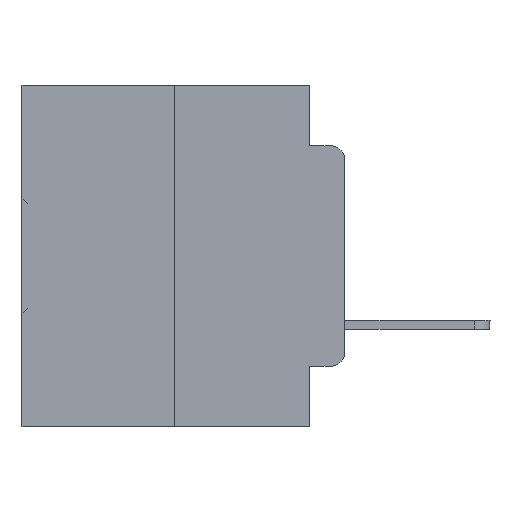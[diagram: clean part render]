
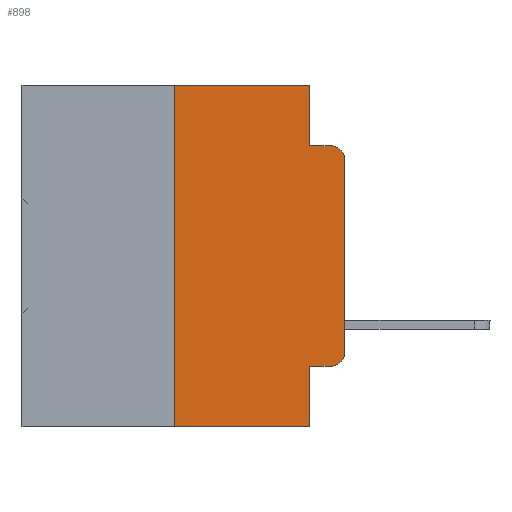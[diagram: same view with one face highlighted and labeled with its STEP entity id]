
A CAD part, left-side view. The second image highlights one B-rep face of the part: STEP entity #898.
In plain terms, the highlighted planar face has unit normal (-1, 0, 0).
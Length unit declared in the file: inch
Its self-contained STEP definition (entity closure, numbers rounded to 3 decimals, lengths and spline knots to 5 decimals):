
#272 = EDGE_CURVE ( 'NONE', #18981, #21185, #23101, .T. ) ;
#529 = DIRECTION ( 'NONE',  ( 0., 0., -1. ) ) ;
#868 = CARTESIAN_POINT ( 'NONE',  ( 0., 0.051, -0.4115 ) ) ;
#898 = ADVANCED_FACE ( 'NONE', ( #8043 ), #26643, .F. ) ;
#2185 = ORIENTED_EDGE ( 'NONE', *, *, #2942, .F. ) ;
#2942 = EDGE_CURVE ( 'NONE', #31427, #11571, #16630, .T. ) ;
#4294 = DIRECTION ( 'NONE',  ( 0., 0., 1. ) ) ;
#5197 = CARTESIAN_POINT ( 'NONE',  ( 0., 0.25, 0. ) ) ;
#5287 = VERTEX_POINT ( 'NONE', #15477 ) ;
#5591 = CARTESIAN_POINT ( 'NONE',  ( 0., 0.051, -0.0885 ) ) ;
#6175 = CARTESIAN_POINT ( 'NONE',  ( 0., 0., 0. ) ) ;
#6260 = LINE ( 'NONE', #33284, #33751 ) ;
#7361 = CARTESIAN_POINT ( 'NONE',  ( 0., 0.051, -0.5 ) ) ;
#7616 = EDGE_CURVE ( 'NONE', #11571, #5287, #29089, .T. ) ;
#7753 = CARTESIAN_POINT ( 'NONE',  ( 0., 0.02, -0.4115 ) ) ;
#7796 = VERTEX_POINT ( 'NONE', #28972 ) ;
#7856 = ORIENTED_EDGE ( 'NONE', *, *, #30176, .F. ) ;
#7921 = CARTESIAN_POINT ( 'NONE',  ( 0., 0.051, -0.0885 ) ) ;
#8043 = FACE_OUTER_BOUND ( 'NONE', #22246, .T. ) ;
#9012 = EDGE_CURVE ( 'NONE', #20275, #7796, #23643, .T. ) ;
#9058 = VECTOR ( 'NONE', #30257, 39.37008 ) ;
#9879 = DIRECTION ( 'NONE',  ( 0., 0., -1. ) ) ;
#9928 = CARTESIAN_POINT ( 'NONE',  ( 0., 0.25, -0.5 ) ) ;
#10040 = CARTESIAN_POINT ( 'NONE',  ( 0., 0.02, -0.1085 ) ) ;
#11191 = VERTEX_POINT ( 'NONE', #7921 ) ;
#11571 = VERTEX_POINT ( 'NONE', #5197 ) ;
#12537 = DIRECTION ( 'NONE',  ( -1., 0., 0. ) ) ;
#12617 = EDGE_CURVE ( 'NONE', #18981, #29494, #6260, .T. ) ;
#12719 = VECTOR ( 'NONE', #9879, 39.37008 ) ;
#13614 = DIRECTION ( 'NONE',  ( 0., -1., 0. ) ) ;
#14363 = DIRECTION ( 'NONE',  ( 0., 0., 1. ) ) ;
#14814 = EDGE_CURVE ( 'NONE', #29494, #20275, #16955, .T. ) ;
#15195 = DIRECTION ( 'NONE',  ( 0., 0., -1. ) ) ;
#15477 = CARTESIAN_POINT ( 'NONE',  ( 0., 0.051, 0. ) ) ;
#15895 = DIRECTION ( 'NONE',  ( 0., -1., 0. ) ) ;
#16044 = LINE ( 'NONE', #30364, #12719 ) ;
#16630 = LINE ( 'NONE', #20285, #24535 ) ;
#16955 = CIRCLE ( 'NONE', #22579, 0.02 ) ;
#17371 = VECTOR ( 'NONE', #13614, 39.37008 ) ;
#17416 = DIRECTION ( 'NONE',  ( 0., -1., 0. ) ) ;
#18526 = ORIENTED_EDGE ( 'NONE', *, *, #14814, .T. ) ;
#18981 = VERTEX_POINT ( 'NONE', #868 ) ;
#19599 = CARTESIAN_POINT ( 'NONE',  ( 0., 0.473, 0. ) ) ;
#20048 = AXIS2_PLACEMENT_3D ( 'NONE', #31523, #34309, #34535 ) ;
#20275 = VERTEX_POINT ( 'NONE', #22421 ) ;
#20285 = CARTESIAN_POINT ( 'NONE',  ( 0., 0.25, 0. ) ) ;
#20353 = EDGE_CURVE ( 'NONE', #7796, #26032, #29438, .T. ) ;
#21185 = VERTEX_POINT ( 'NONE', #7361 ) ;
#21705 = ORIENTED_EDGE ( 'NONE', *, *, #27758, .T. ) ;
#21818 = CARTESIAN_POINT ( 'NONE',  ( 0., 0.02, -0.3915 ) ) ;
#21957 = EDGE_CURVE ( 'NONE', #5287, #11191, #16044, .T. ) ;
#22161 = DIRECTION ( 'NONE',  ( -1., 0., 0. ) ) ;
#22246 = EDGE_LOOP ( 'NONE', ( #31153, #28973, #7856, #29403, #27926, #2185, #21705, #22296, #26264, #18526 ) ) ;
#22296 = ORIENTED_EDGE ( 'NONE', *, *, #272, .F. ) ;
#22421 = CARTESIAN_POINT ( 'NONE',  ( 0., 0., -0.3915 ) ) ;
#22579 = AXIS2_PLACEMENT_3D ( 'NONE', #21818, #22161, #529 ) ;
#22809 = LINE ( 'NONE', #5591, #27746 ) ;
#23101 = LINE ( 'NONE', #31452, #32966 ) ;
#23643 = LINE ( 'NONE', #6175, #33560 ) ;
#24535 = VECTOR ( 'NONE', #4294, 39.37008 ) ;
#26032 = VERTEX_POINT ( 'NONE', #28957 ) ;
#26264 = ORIENTED_EDGE ( 'NONE', *, *, #12617, .T. ) ;
#26643 = PLANE ( 'NONE',  #20048 ) ;
#27746 = VECTOR ( 'NONE', #15895, 39.37008 ) ;
#27758 = EDGE_CURVE ( 'NONE', #31427, #21185, #30239, .T. ) ;
#27926 = ORIENTED_EDGE ( 'NONE', *, *, #7616, .F. ) ;
#28957 = CARTESIAN_POINT ( 'NONE',  ( 0., 0.02, -0.0885 ) ) ;
#28973 = ORIENTED_EDGE ( 'NONE', *, *, #20353, .T. ) ;
#28972 = CARTESIAN_POINT ( 'NONE',  ( 0., 0., -0.1085 ) ) ;
#29089 = LINE ( 'NONE', #19599, #9058 ) ;
#29403 = ORIENTED_EDGE ( 'NONE', *, *, #21957, .F. ) ;
#29438 = CIRCLE ( 'NONE', #32089, 0.02 ) ;
#29494 = VERTEX_POINT ( 'NONE', #7753 ) ;
#29500 = CARTESIAN_POINT ( 'NONE',  ( 0., 0.473, -0.5 ) ) ;
#30176 = EDGE_CURVE ( 'NONE', #11191, #26032, #22809, .T. ) ;
#30239 = LINE ( 'NONE', #29500, #17371 ) ;
#30257 = DIRECTION ( 'NONE',  ( 0., -1., 0. ) ) ;
#30364 = CARTESIAN_POINT ( 'NONE',  ( 0., 0.051, 0. ) ) ;
#31153 = ORIENTED_EDGE ( 'NONE', *, *, #9012, .T. ) ;
#31427 = VERTEX_POINT ( 'NONE', #9928 ) ;
#31452 = CARTESIAN_POINT ( 'NONE',  ( 0., 0.051, 0. ) ) ;
#31523 = CARTESIAN_POINT ( 'NONE',  ( 0., 0.473, 0. ) ) ;
#32089 = AXIS2_PLACEMENT_3D ( 'NONE', #10040, #12537, #15195 ) ;
#32966 = VECTOR ( 'NONE', #34126, 39.37008 ) ;
#33284 = CARTESIAN_POINT ( 'NONE',  ( 0., 0.051, -0.4115 ) ) ;
#33560 = VECTOR ( 'NONE', #14363, 39.37008 ) ;
#33751 = VECTOR ( 'NONE', #17416, 39.37008 ) ;
#34126 = DIRECTION ( 'NONE',  ( 0., 0., -1. ) ) ;
#34309 = DIRECTION ( 'NONE',  ( 1., 0., 0. ) ) ;
#34535 = DIRECTION ( 'NONE',  ( 0., 0., -1. ) ) ;
